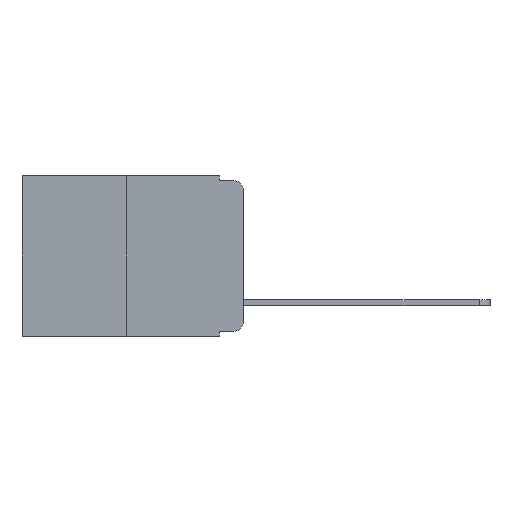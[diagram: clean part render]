
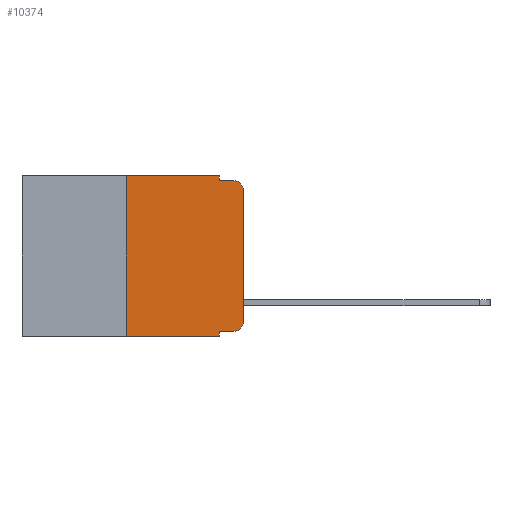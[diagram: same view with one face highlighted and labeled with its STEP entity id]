
A CAD part, left-side view. The second image highlights one B-rep face of the part: STEP entity #10374.
In plain terms, the highlighted planar face has unit normal (-1, 0, 0).
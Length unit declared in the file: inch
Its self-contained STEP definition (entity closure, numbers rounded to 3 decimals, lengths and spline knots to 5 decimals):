
#11 = DIRECTION ( 'NONE',  ( 1., 0., 0. ) ) ;
#167 = CARTESIAN_POINT ( 'NONE',  ( 0., 0., 0. ) ) ;
#321 = LINE ( 'NONE', #15331, #14359 ) ;
#390 = CARTESIAN_POINT ( 'NONE',  ( 0., 0.051, -0.333 ) ) ;
#551 = CARTESIAN_POINT ( 'NONE',  ( 0., 0.25, 0. ) ) ;
#741 = LINE ( 'NONE', #12925, #14722 ) ;
#856 = CARTESIAN_POINT ( 'NONE',  ( 0., 0.02, -0.03 ) ) ;
#969 = EDGE_CURVE ( 'NONE', #11152, #7530, #4729, .T. ) ;
#1108 = VERTEX_POINT ( 'NONE', #14687 ) ;
#1133 = LINE ( 'NONE', #5691, #15057 ) ;
#1224 = EDGE_CURVE ( 'NONE', #7530, #6558, #741, .T. ) ;
#1618 = DIRECTION ( 'NONE',  ( -1., 0., 0. ) ) ;
#1755 = CARTESIAN_POINT ( 'NONE',  ( 0., 0.473, 0. ) ) ;
#2127 = VECTOR ( 'NONE', #9982, 39.37008 ) ;
#2141 = ORIENTED_EDGE ( 'NONE', *, *, #969, .F. ) ;
#2295 = DIRECTION ( 'NONE',  ( 0., 0., -1. ) ) ;
#2402 = CARTESIAN_POINT ( 'NONE',  ( 0., 0.02, -0.333 ) ) ;
#2426 = EDGE_CURVE ( 'NONE', #11697, #1108, #12565, .T. ) ;
#3374 = CARTESIAN_POINT ( 'NONE',  ( 0., 0.051, 0. ) ) ;
#3570 = VERTEX_POINT ( 'NONE', #390 ) ;
#3761 = VERTEX_POINT ( 'NONE', #8307 ) ;
#3981 = FACE_OUTER_BOUND ( 'NONE', #10589, .T. ) ;
#4146 = ORIENTED_EDGE ( 'NONE', *, *, #2426, .T. ) ;
#4245 = PLANE ( 'NONE',  #5272 ) ;
#4702 = DIRECTION ( 'NONE',  ( 0., 0., -1. ) ) ;
#4729 = LINE ( 'NONE', #8187, #14929 ) ;
#5220 = ORIENTED_EDGE ( 'NONE', *, *, #11830, .T. ) ;
#5272 = AXIS2_PLACEMENT_3D ( 'NONE', #8337, #11, #9696 ) ;
#5435 = VECTOR ( 'NONE', #12390, 39.37008 ) ;
#5691 = CARTESIAN_POINT ( 'NONE',  ( 0., 0.473, -0.343 ) ) ;
#6558 = VERTEX_POINT ( 'NONE', #16004 ) ;
#7121 = ORIENTED_EDGE ( 'NONE', *, *, #17297, .T. ) ;
#7250 = VERTEX_POINT ( 'NONE', #8561 ) ;
#7530 = VERTEX_POINT ( 'NONE', #9081 ) ;
#8187 = CARTESIAN_POINT ( 'NONE',  ( 0., 0.051, 0. ) ) ;
#8190 = ORIENTED_EDGE ( 'NONE', *, *, #9521, .T. ) ;
#8307 = CARTESIAN_POINT ( 'NONE',  ( 0., 0.051, -0.343 ) ) ;
#8337 = CARTESIAN_POINT ( 'NONE',  ( 0., 0.473, 0. ) ) ;
#8561 = CARTESIAN_POINT ( 'NONE',  ( 0., 0.25, -0.343 ) ) ;
#8792 = VERTEX_POINT ( 'NONE', #551 ) ;
#9081 = CARTESIAN_POINT ( 'NONE',  ( 0., 0.051, -0.01 ) ) ;
#9431 = LINE ( 'NONE', #1755, #2127 ) ;
#9521 = EDGE_CURVE ( 'NONE', #1108, #6558, #16432, .T. ) ;
#9696 = DIRECTION ( 'NONE',  ( 0., 0., -1. ) ) ;
#9847 = CARTESIAN_POINT ( 'NONE',  ( 0., 0.02, -0.313 ) ) ;
#9871 = CARTESIAN_POINT ( 'NONE',  ( 0., 0., -0.313 ) ) ;
#9982 = DIRECTION ( 'NONE',  ( 0., -1., 0. ) ) ;
#10374 = ADVANCED_FACE ( 'NONE', ( #3981 ), #4245, .F. ) ;
#10452 = VECTOR ( 'NONE', #12278, 39.37008 ) ;
#10484 = DIRECTION ( 'NONE',  ( -1., 0., 0. ) ) ;
#10589 = EDGE_LOOP ( 'NONE', ( #4146, #8190, #15177, #2141, #16763, #17167, #7121, #11113, #5220, #16175 ) ) ;
#10866 = LINE ( 'NONE', #16165, #10452 ) ;
#10997 = AXIS2_PLACEMENT_3D ( 'NONE', #9847, #1618, #11168 ) ;
#11113 = ORIENTED_EDGE ( 'NONE', *, *, #13589, .F. ) ;
#11152 = VERTEX_POINT ( 'NONE', #3374 ) ;
#11168 = DIRECTION ( 'NONE',  ( 0., 0., -1. ) ) ;
#11187 = DIRECTION ( 'NONE',  ( 0., 0., -1. ) ) ;
#11697 = VERTEX_POINT ( 'NONE', #9871 ) ;
#11740 = VECTOR ( 'NONE', #4702, 39.37008 ) ;
#11751 = EDGE_CURVE ( 'NONE', #8792, #11152, #9431, .T. ) ;
#11830 = EDGE_CURVE ( 'NONE', #3570, #16777, #321, .T. ) ;
#12004 = AXIS2_PLACEMENT_3D ( 'NONE', #856, #10484, #2295 ) ;
#12278 = DIRECTION ( 'NONE',  ( 0., 0., 1. ) ) ;
#12390 = DIRECTION ( 'NONE',  ( 0., 0., 1. ) ) ;
#12565 = LINE ( 'NONE', #167, #5435 ) ;
#12925 = CARTESIAN_POINT ( 'NONE',  ( 0., 0.051, -0.01 ) ) ;
#12976 = LINE ( 'NONE', #16552, #11740 ) ;
#13589 = EDGE_CURVE ( 'NONE', #3570, #3761, #12976, .T. ) ;
#13692 = DIRECTION ( 'NONE',  ( 0., -1., 0. ) ) ;
#14359 = VECTOR ( 'NONE', #16606, 39.37008 ) ;
#14610 = DIRECTION ( 'NONE',  ( 0., -1., 0. ) ) ;
#14655 = CIRCLE ( 'NONE', #10997, 0.02 ) ;
#14687 = CARTESIAN_POINT ( 'NONE',  ( 0., 0., -0.03 ) ) ;
#14722 = VECTOR ( 'NONE', #14610, 39.37008 ) ;
#14929 = VECTOR ( 'NONE', #11187, 39.37008 ) ;
#15057 = VECTOR ( 'NONE', #13692, 39.37008 ) ;
#15177 = ORIENTED_EDGE ( 'NONE', *, *, #1224, .F. ) ;
#15304 = EDGE_CURVE ( 'NONE', #7250, #8792, #10866, .T. ) ;
#15331 = CARTESIAN_POINT ( 'NONE',  ( 0., 0.051, -0.333 ) ) ;
#16004 = CARTESIAN_POINT ( 'NONE',  ( 0., 0.02, -0.01 ) ) ;
#16165 = CARTESIAN_POINT ( 'NONE',  ( 0., 0.25, 0. ) ) ;
#16175 = ORIENTED_EDGE ( 'NONE', *, *, #17324, .T. ) ;
#16432 = CIRCLE ( 'NONE', #12004, 0.02 ) ;
#16552 = CARTESIAN_POINT ( 'NONE',  ( 0., 0.051, 0. ) ) ;
#16606 = DIRECTION ( 'NONE',  ( 0., -1., 0. ) ) ;
#16763 = ORIENTED_EDGE ( 'NONE', *, *, #11751, .F. ) ;
#16777 = VERTEX_POINT ( 'NONE', #2402 ) ;
#17167 = ORIENTED_EDGE ( 'NONE', *, *, #15304, .F. ) ;
#17297 = EDGE_CURVE ( 'NONE', #7250, #3761, #1133, .T. ) ;
#17324 = EDGE_CURVE ( 'NONE', #16777, #11697, #14655, .T. ) ;
